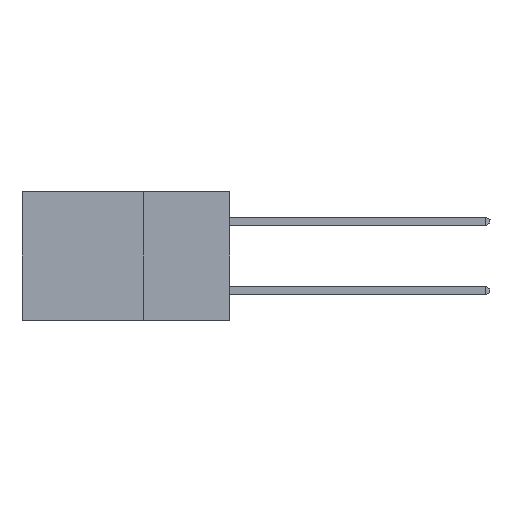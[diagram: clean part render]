
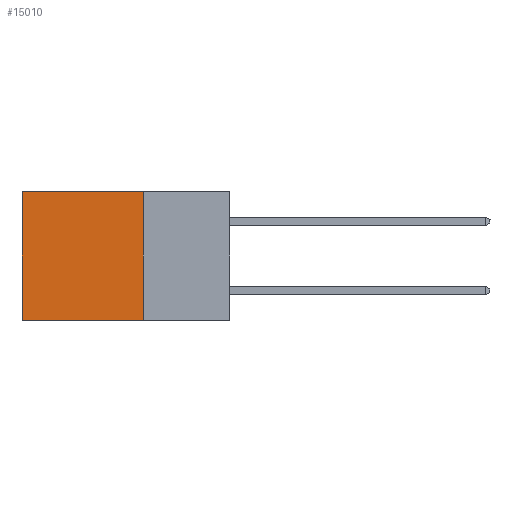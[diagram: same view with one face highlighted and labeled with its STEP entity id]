
A CAD part, left-side view. The second image highlights one B-rep face of the part: STEP entity #15010.
In plain terms, the highlighted planar face has unit normal (-1, 0, 0).
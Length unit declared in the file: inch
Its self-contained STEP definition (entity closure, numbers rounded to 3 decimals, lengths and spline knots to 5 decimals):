
#313 = CARTESIAN_POINT ( 'NONE',  ( 0.298, 0.25, 0. ) ) ;
#1153 = EDGE_CURVE ( 'NONE', #13222, #10431, #7566, .T. ) ;
#1355 = VERTEX_POINT ( 'NONE', #12282 ) ;
#1503 = VERTEX_POINT ( 'NONE', #13874 ) ;
#1656 = LINE ( 'NONE', #2946, #4928 ) ;
#2755 = ORIENTED_EDGE ( 'NONE', *, *, #14179, .T. ) ;
#2946 = CARTESIAN_POINT ( 'NONE',  ( 0.298, 0.6, 0. ) ) ;
#3736 = CARTESIAN_POINT ( 'NONE',  ( 0.298, 0.25, -0.37 ) ) ;
#4455 = LINE ( 'NONE', #3736, #5893 ) ;
#4928 = VECTOR ( 'NONE', #6733, 39.37008 ) ;
#5027 = EDGE_CURVE ( 'NONE', #1355, #1503, #1656, .T. ) ;
#5281 = EDGE_LOOP ( 'NONE', ( #12108, #15173, #13061, #2755 ) ) ;
#5432 = LINE ( 'NONE', #6539, #7280 ) ;
#5643 = PLANE ( 'NONE',  #16645 ) ;
#5893 = VECTOR ( 'NONE', #8916, 39.37008 ) ;
#6539 = CARTESIAN_POINT ( 'NONE',  ( 0.298, 0.25, 0. ) ) ;
#6733 = DIRECTION ( 'NONE',  ( 0., 0., -1. ) ) ;
#7280 = VECTOR ( 'NONE', #7967, 39.37008 ) ;
#7566 = LINE ( 'NONE', #7815, #10435 ) ;
#7815 = CARTESIAN_POINT ( 'NONE',  ( 0.298, 0.25, 0. ) ) ;
#7967 = DIRECTION ( 'NONE',  ( 0., 1., 0. ) ) ;
#8342 = DIRECTION ( 'NONE',  ( 0., 0., -1. ) ) ;
#8676 = CARTESIAN_POINT ( 'NONE',  ( 0.298, 0.25, 0. ) ) ;
#8916 = DIRECTION ( 'NONE',  ( 0., 1., 0. ) ) ;
#10431 = VERTEX_POINT ( 'NONE', #14615 ) ;
#10435 = VECTOR ( 'NONE', #11684, 39.37008 ) ;
#11684 = DIRECTION ( 'NONE',  ( 0., 0., -1. ) ) ;
#12108 = ORIENTED_EDGE ( 'NONE', *, *, #5027, .T. ) ;
#12282 = CARTESIAN_POINT ( 'NONE',  ( 0.298, 0.6, 0. ) ) ;
#13061 = ORIENTED_EDGE ( 'NONE', *, *, #1153, .F. ) ;
#13222 = VERTEX_POINT ( 'NONE', #8676 ) ;
#13497 = FACE_OUTER_BOUND ( 'NONE', #5281, .T. ) ;
#13606 = DIRECTION ( 'NONE',  ( 1., 0., 0. ) ) ;
#13874 = CARTESIAN_POINT ( 'NONE',  ( 0.298, 0.6, -0.37 ) ) ;
#14179 = EDGE_CURVE ( 'NONE', #13222, #1355, #5432, .T. ) ;
#14615 = CARTESIAN_POINT ( 'NONE',  ( 0.298, 0.25, -0.37 ) ) ;
#14853 = EDGE_CURVE ( 'NONE', #10431, #1503, #4455, .T. ) ;
#15010 = ADVANCED_FACE ( 'NONE', ( #13497 ), #5643, .F. ) ;
#15173 = ORIENTED_EDGE ( 'NONE', *, *, #14853, .F. ) ;
#16645 = AXIS2_PLACEMENT_3D ( 'NONE', #313, #13606, #8342 ) ;
